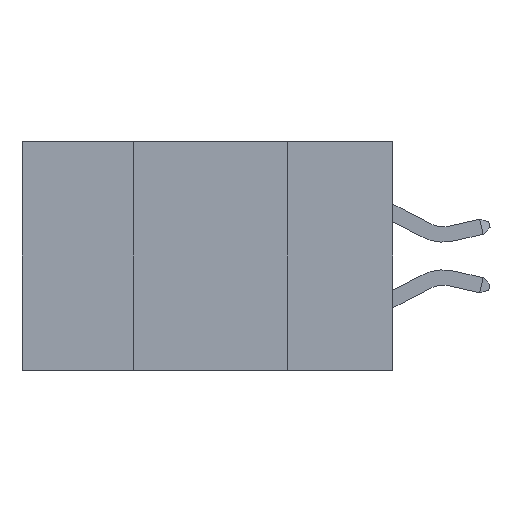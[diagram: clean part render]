
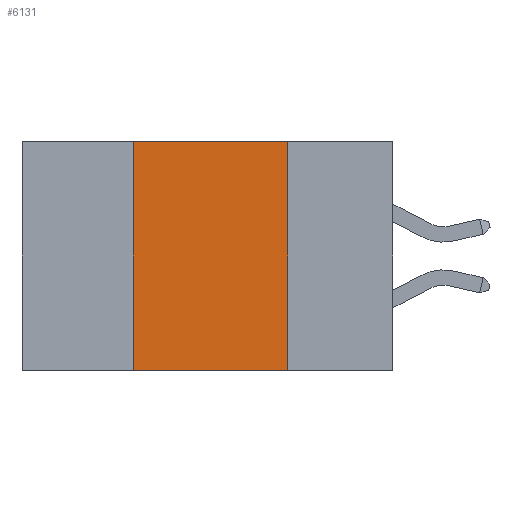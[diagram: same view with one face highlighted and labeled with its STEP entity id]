
A CAD part, left-side view. The second image highlights one B-rep face of the part: STEP entity #6131.
In plain terms, the highlighted planar face has unit normal (-1, 0, 0).
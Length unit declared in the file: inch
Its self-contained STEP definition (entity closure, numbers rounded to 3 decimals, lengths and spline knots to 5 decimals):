
#1370 = VERTEX_POINT ( 'NONE', #21338 ) ;
#1935 = CARTESIAN_POINT ( 'NONE',  ( 0., 0.42, 0. ) ) ;
#2882 = CARTESIAN_POINT ( 'NONE',  ( 0., 0.6, -0.37 ) ) ;
#5040 = ORIENTED_EDGE ( 'NONE', *, *, #32411, .F. ) ;
#5479 = CARTESIAN_POINT ( 'NONE',  ( 0., 0.17, 0. ) ) ;
#6131 = ADVANCED_FACE ( 'NONE', ( #13302 ), #16615, .F. ) ;
#6197 = DIRECTION ( 'NONE',  ( 0., -1., 0. ) ) ;
#7979 = DIRECTION ( 'NONE',  ( 0., 0., 1. ) ) ;
#8968 = AXIS2_PLACEMENT_3D ( 'NONE', #13687, #16034, #21829 ) ;
#10122 = EDGE_CURVE ( 'NONE', #19808, #29157, #37300, .T. ) ;
#10278 = ORIENTED_EDGE ( 'NONE', *, *, #10122, .F. ) ;
#10804 = EDGE_CURVE ( 'NONE', #1370, #29157, #27143, .T. ) ;
#13302 = FACE_OUTER_BOUND ( 'NONE', #36851, .T. ) ;
#13534 = LINE ( 'NONE', #15665, #14995 ) ;
#13687 = CARTESIAN_POINT ( 'NONE',  ( 0., 0.6, 0. ) ) ;
#14504 = CARTESIAN_POINT ( 'NONE',  ( 0., 0.42, 0. ) ) ;
#14995 = VECTOR ( 'NONE', #28262, 39.37008 ) ;
#15665 = CARTESIAN_POINT ( 'NONE',  ( 0., 0.6, 0. ) ) ;
#16034 = DIRECTION ( 'NONE',  ( 1., 0., 0. ) ) ;
#16550 = ORIENTED_EDGE ( 'NONE', *, *, #17482, .F. ) ;
#16615 = PLANE ( 'NONE',  #8968 ) ;
#17366 = VECTOR ( 'NONE', #7979, 39.37008 ) ;
#17482 = EDGE_CURVE ( 'NONE', #24723, #19808, #13534, .T. ) ;
#17611 = VECTOR ( 'NONE', #31499, 39.37008 ) ;
#19808 = VERTEX_POINT ( 'NONE', #29101 ) ;
#21338 = CARTESIAN_POINT ( 'NONE',  ( 0., 0.42, -0.37 ) ) ;
#21829 = DIRECTION ( 'NONE',  ( 0., 0., -1. ) ) ;
#24723 = VERTEX_POINT ( 'NONE', #14504 ) ;
#25095 = VECTOR ( 'NONE', #6197, 39.37008 ) ;
#27143 = LINE ( 'NONE', #2882, #25095 ) ;
#28262 = DIRECTION ( 'NONE',  ( 0., -1., 0. ) ) ;
#28301 = ORIENTED_EDGE ( 'NONE', *, *, #10804, .T. ) ;
#28531 = LINE ( 'NONE', #1935, #17366 ) ;
#29101 = CARTESIAN_POINT ( 'NONE',  ( 0., 0.17, 0. ) ) ;
#29157 = VERTEX_POINT ( 'NONE', #30662 ) ;
#30662 = CARTESIAN_POINT ( 'NONE',  ( 0., 0.17, -0.37 ) ) ;
#31499 = DIRECTION ( 'NONE',  ( 0., 0., -1. ) ) ;
#32411 = EDGE_CURVE ( 'NONE', #1370, #24723, #28531, .T. ) ;
#36851 = EDGE_LOOP ( 'NONE', ( #10278, #16550, #5040, #28301 ) ) ;
#37300 = LINE ( 'NONE', #5479, #17611 ) ;
